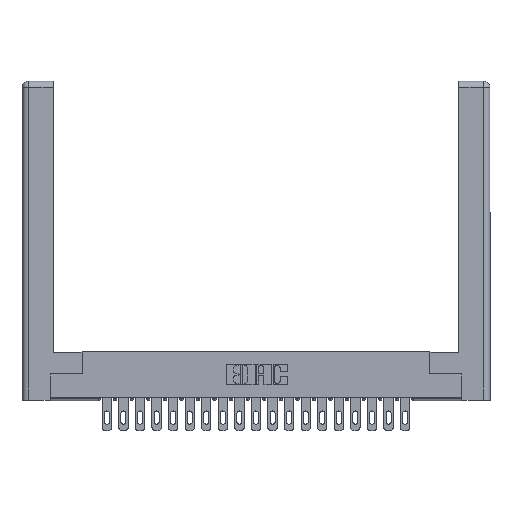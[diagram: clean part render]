
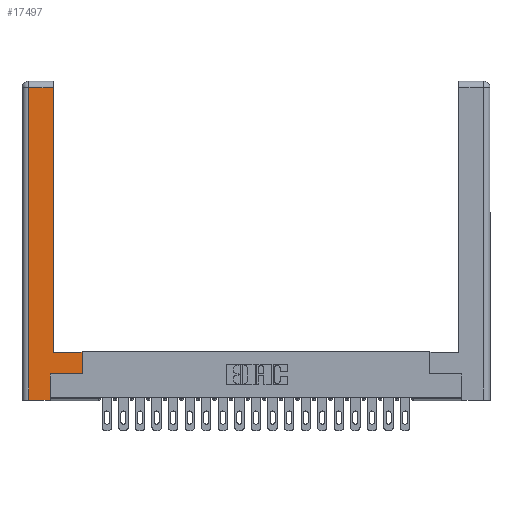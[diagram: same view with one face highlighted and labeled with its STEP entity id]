
A CAD part, top view. The second image highlights one B-rep face of the part: STEP entity #17497.
In plain terms, the highlighted planar face has unit normal (0, 0, 1).
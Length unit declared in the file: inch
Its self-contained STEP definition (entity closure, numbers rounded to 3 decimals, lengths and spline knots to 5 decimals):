
#66 = LINE ( 'NONE', #21615, #12088 ) ;
#108 = DIRECTION ( 'NONE',  ( 0., 1., 0. ) ) ;
#244 = ORIENTED_EDGE ( 'NONE', *, *, #1182, .T. ) ;
#1039 = DIRECTION ( 'NONE',  ( 0., 1., 0. ) ) ;
#1182 = EDGE_CURVE ( 'NONE', #13266, #22780, #22262, .T. ) ;
#1242 = VECTOR ( 'NONE', #17099, 39.37008 ) ;
#1401 = ORIENTED_EDGE ( 'NONE', *, *, #16890, .T. ) ;
#1677 = PLANE ( 'NONE',  #9202 ) ;
#2089 = DIRECTION ( 'NONE',  ( 1., 0., 0. ) ) ;
#2955 = CARTESIAN_POINT ( 'NONE',  ( 0.565, 0.245, 0. ) ) ;
#3195 = CARTESIAN_POINT ( 'NONE',  ( 0.265, 0., 0. ) ) ;
#3313 = ORIENTED_EDGE ( 'NONE', *, *, #10933, .T. ) ;
#3357 = LINE ( 'NONE', #23336, #13129 ) ;
#3673 = LINE ( 'NONE', #16392, #22463 ) ;
#4063 = VERTEX_POINT ( 'NONE', #11900 ) ;
#4231 = CARTESIAN_POINT ( 'NONE',  ( 0.265, 0.245, 0. ) ) ;
#4349 = VERTEX_POINT ( 'NONE', #11515 ) ;
#5256 = CARTESIAN_POINT ( 'NONE',  ( 0., 0., 0. ) ) ;
#6536 = VECTOR ( 'NONE', #13810, 39.37008 ) ;
#6646 = EDGE_CURVE ( 'NONE', #22780, #9473, #3357, .T. ) ;
#6801 = DIRECTION ( 'NONE',  ( -1., 0., 0. ) ) ;
#7016 = ORIENTED_EDGE ( 'NONE', *, *, #17593, .T. ) ;
#7311 = DIRECTION ( 'NONE',  ( -1., 0., 0. ) ) ;
#7378 = VERTEX_POINT ( 'NONE', #2955 ) ;
#7597 = LINE ( 'NONE', #13063, #1242 ) ;
#7756 = CARTESIAN_POINT ( 'NONE',  ( 0.295, 0.45, 0. ) ) ;
#7892 = CARTESIAN_POINT ( 'NONE',  ( 0.265, 0., 0. ) ) ;
#9195 = EDGE_CURVE ( 'NONE', #4349, #13266, #66, .T. ) ;
#9202 = AXIS2_PLACEMENT_3D ( 'NONE', #5256, #10242, #15956 ) ;
#9473 = VERTEX_POINT ( 'NONE', #22810 ) ;
#9792 = LINE ( 'NONE', #19207, #20475 ) ;
#9906 = DIRECTION ( 'NONE',  ( 0., 1., 0. ) ) ;
#10242 = DIRECTION ( 'NONE',  ( 0., 0., -1. ) ) ;
#10884 = VERTEX_POINT ( 'NONE', #4231 ) ;
#10933 = EDGE_CURVE ( 'NONE', #10884, #7378, #11020, .T. ) ;
#10982 = EDGE_CURVE ( 'NONE', #19756, #10884, #9792, .T. ) ;
#11020 = LINE ( 'NONE', #16483, #11728 ) ;
#11515 = CARTESIAN_POINT ( 'NONE',  ( 0.565, 0.45, 0. ) ) ;
#11728 = VECTOR ( 'NONE', #2089, 39.37008 ) ;
#11900 = CARTESIAN_POINT ( 'NONE',  ( 0.0615, 0., 0. ) ) ;
#12088 = VECTOR ( 'NONE', #7311, 39.37008 ) ;
#12125 = LINE ( 'NONE', #3195, #6536 ) ;
#13063 = CARTESIAN_POINT ( 'NONE',  ( 0.0615, 0., 0. ) ) ;
#13129 = VECTOR ( 'NONE', #6801, 39.37008 ) ;
#13266 = VERTEX_POINT ( 'NONE', #7756 ) ;
#13356 = VECTOR ( 'NONE', #1039, 39.37008 ) ;
#13810 = DIRECTION ( 'NONE',  ( 1., 0., 0. ) ) ;
#13887 = EDGE_LOOP ( 'NONE', ( #244, #20734, #7016, #1401, #22124, #3313, #15303, #15587 ) ) ;
#15093 = EDGE_CURVE ( 'NONE', #7378, #4349, #3673, .T. ) ;
#15303 = ORIENTED_EDGE ( 'NONE', *, *, #15093, .T. ) ;
#15587 = ORIENTED_EDGE ( 'NONE', *, *, #9195, .T. ) ;
#15956 = DIRECTION ( 'NONE',  ( -1., 0., 0. ) ) ;
#16392 = CARTESIAN_POINT ( 'NONE',  ( 0.565, 0.45, 0. ) ) ;
#16483 = CARTESIAN_POINT ( 'NONE',  ( 0.565, 0.245, 0. ) ) ;
#16856 = CARTESIAN_POINT ( 'NONE',  ( 0.295, 2.94, 0. ) ) ;
#16890 = EDGE_CURVE ( 'NONE', #4063, #19756, #12125, .T. ) ;
#17099 = DIRECTION ( 'NONE',  ( 0., -1., 0. ) ) ;
#17497 = ADVANCED_FACE ( 'NONE', ( #22986 ), #1677, .F. ) ;
#17593 = EDGE_CURVE ( 'NONE', #9473, #4063, #7597, .T. ) ;
#19207 = CARTESIAN_POINT ( 'NONE',  ( 0.265, 0.245, 0. ) ) ;
#19756 = VERTEX_POINT ( 'NONE', #7892 ) ;
#20475 = VECTOR ( 'NONE', #9906, 39.37008 ) ;
#20734 = ORIENTED_EDGE ( 'NONE', *, *, #6646, .T. ) ;
#20927 = CARTESIAN_POINT ( 'NONE',  ( 0.295, 3., 0. ) ) ;
#21615 = CARTESIAN_POINT ( 'NONE',  ( 0.295, 0.45, 0. ) ) ;
#22124 = ORIENTED_EDGE ( 'NONE', *, *, #10982, .T. ) ;
#22262 = LINE ( 'NONE', #20927, #13356 ) ;
#22463 = VECTOR ( 'NONE', #108, 39.37008 ) ;
#22780 = VERTEX_POINT ( 'NONE', #16856 ) ;
#22810 = CARTESIAN_POINT ( 'NONE',  ( 0.0615, 2.94, 0. ) ) ;
#22986 = FACE_OUTER_BOUND ( 'NONE', #13887, .T. ) ;
#23336 = CARTESIAN_POINT ( 'NONE',  ( 0.0615, 2.94, 0. ) ) ;
